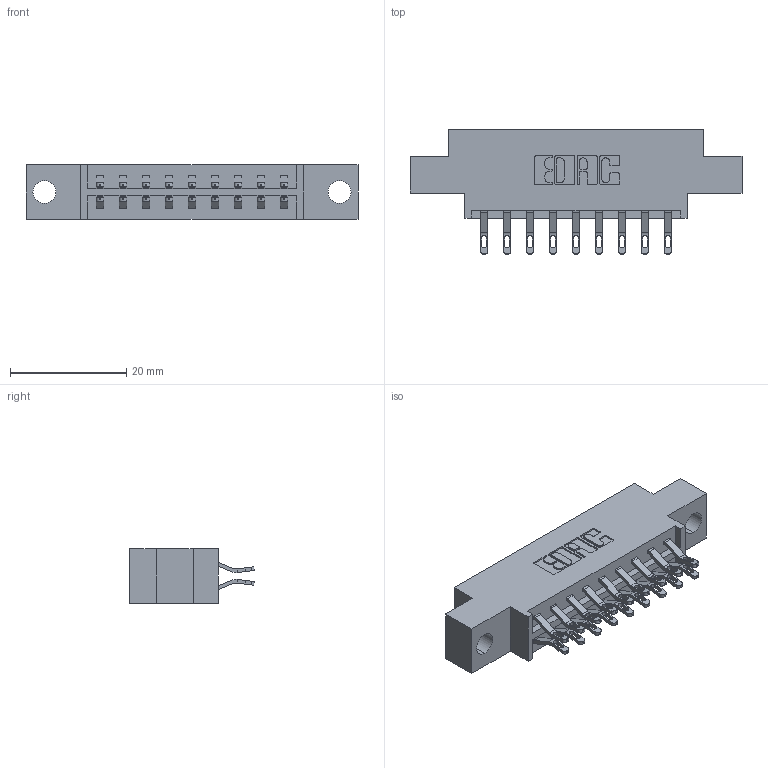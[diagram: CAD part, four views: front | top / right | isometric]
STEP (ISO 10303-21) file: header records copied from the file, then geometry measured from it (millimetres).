
FILE_DESCRIPTION (( 'STEP AP203' ), '1' );
FILE_NAME ('833-018-555-804.STEP', '2020-05-31T22:58:48', ( '' ), ( '' ), 'SwSTEP 2.0', 'SolidWorks 2020', '' );
FILE_SCHEMA (( 'CONFIG_CONTROL_DESIGN' ));
Length unit declared in the file: inch
Products named in the file (3): 833-018-555-804; 345-292-001_555 Tail; 833 Part_Offset - .156 Dia - TH
Assembly tree (19 placements, depth 2):
  833-018-555-804
    833 Part_Offset - .156 Dia - TH
    345-292-001_555 Tail  x18
Bounding box: 57.2 x 21.47 x 9.4 mm (x, y, z)
Volume: 5267.8 mm3; surface area: 6088.8 mm2
Topology: 19 solids, 19 shells, 1162 faces, 3617 edges, 2410 vertices
Faces by surface type: plane 686, cylinder 476
Entity records: 10519 total; most frequent: CARTESIAN_POINT 1820, ORIENTED_EDGE 1726, DIRECTION 1583, EDGE_CURVE 863, VECTOR 715, LINE 715, VERTEX_POINT 574, AXIS2_PLACEMENT_3D 434
